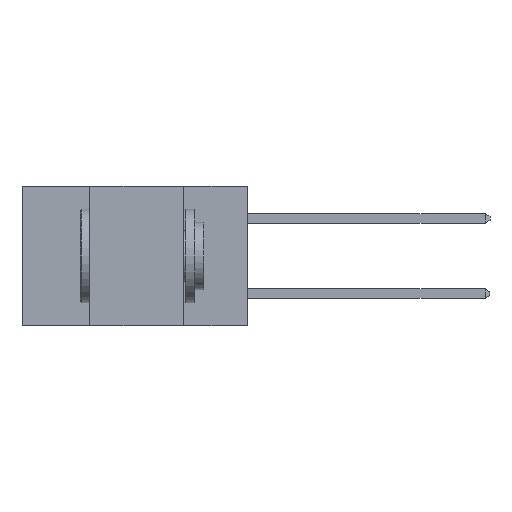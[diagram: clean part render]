
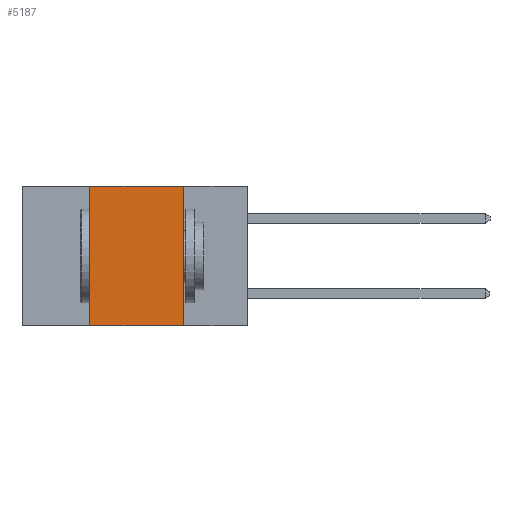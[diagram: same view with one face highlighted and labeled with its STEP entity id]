
A CAD part, left-side view. The second image highlights one B-rep face of the part: STEP entity #5187.
In plain terms, the highlighted planar face has unit normal (-1, 0, 0).
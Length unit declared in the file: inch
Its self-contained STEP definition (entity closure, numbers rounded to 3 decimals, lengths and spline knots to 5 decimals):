
#126 = ORIENTED_EDGE ( 'NONE', *, *, #12302, .F. ) ;
#170 = CARTESIAN_POINT ( 'NONE',  ( 0., 0.42, 0. ) ) ;
#210 = ORIENTED_EDGE ( 'NONE', *, *, #6367, .F. ) ;
#1208 = VERTEX_POINT ( 'NONE', #8634 ) ;
#1824 = DIRECTION ( 'NONE',  ( 0., -1., 0. ) ) ;
#2518 = LINE ( 'NONE', #7133, #12595 ) ;
#3197 = VERTEX_POINT ( 'NONE', #11984 ) ;
#3241 = CARTESIAN_POINT ( 'NONE',  ( 0., 0.42, 0. ) ) ;
#3915 = LINE ( 'NONE', #8747, #9153 ) ;
#4451 = DIRECTION ( 'NONE',  ( 0., 0., -1. ) ) ;
#4896 = EDGE_LOOP ( 'NONE', ( #6932, #126, #210, #10071 ) ) ;
#5001 = VERTEX_POINT ( 'NONE', #11783 ) ;
#5187 = ADVANCED_FACE ( 'NONE', ( #12652 ), #10485, .F. ) ;
#6367 = EDGE_CURVE ( 'NONE', #1208, #9040, #9628, .T. ) ;
#6932 = ORIENTED_EDGE ( 'NONE', *, *, #12084, .F. ) ;
#7133 = CARTESIAN_POINT ( 'NONE',  ( 0., 0.6, -0.37 ) ) ;
#7424 = EDGE_CURVE ( 'NONE', #1208, #5001, #2518, .T. ) ;
#8180 = CARTESIAN_POINT ( 'NONE',  ( 0., 0.6, 0. ) ) ;
#8381 = DIRECTION ( 'NONE',  ( 0., -1., 0. ) ) ;
#8634 = CARTESIAN_POINT ( 'NONE',  ( 0., 0.42, -0.37 ) ) ;
#8747 = CARTESIAN_POINT ( 'NONE',  ( 0., 0.6, 0. ) ) ;
#9001 = VECTOR ( 'NONE', #4451, 39.37008 ) ;
#9040 = VERTEX_POINT ( 'NONE', #170 ) ;
#9153 = VECTOR ( 'NONE', #1824, 39.37008 ) ;
#9628 = LINE ( 'NONE', #3241, #11906 ) ;
#10071 = ORIENTED_EDGE ( 'NONE', *, *, #7424, .T. ) ;
#10485 = PLANE ( 'NONE',  #10791 ) ;
#10791 = AXIS2_PLACEMENT_3D ( 'NONE', #8180, #11681, #11671 ) ;
#11315 = CARTESIAN_POINT ( 'NONE',  ( 0., 0.17, 0. ) ) ;
#11542 = DIRECTION ( 'NONE',  ( 0., 0., 1. ) ) ;
#11671 = DIRECTION ( 'NONE',  ( 0., 0., -1. ) ) ;
#11681 = DIRECTION ( 'NONE',  ( 1., 0., 0. ) ) ;
#11783 = CARTESIAN_POINT ( 'NONE',  ( 0., 0.17, -0.37 ) ) ;
#11899 = LINE ( 'NONE', #11315, #9001 ) ;
#11906 = VECTOR ( 'NONE', #11542, 39.37008 ) ;
#11984 = CARTESIAN_POINT ( 'NONE',  ( 0., 0.17, 0. ) ) ;
#12084 = EDGE_CURVE ( 'NONE', #3197, #5001, #11899, .T. ) ;
#12302 = EDGE_CURVE ( 'NONE', #9040, #3197, #3915, .T. ) ;
#12595 = VECTOR ( 'NONE', #8381, 39.37008 ) ;
#12652 = FACE_OUTER_BOUND ( 'NONE', #4896, .T. ) ;
